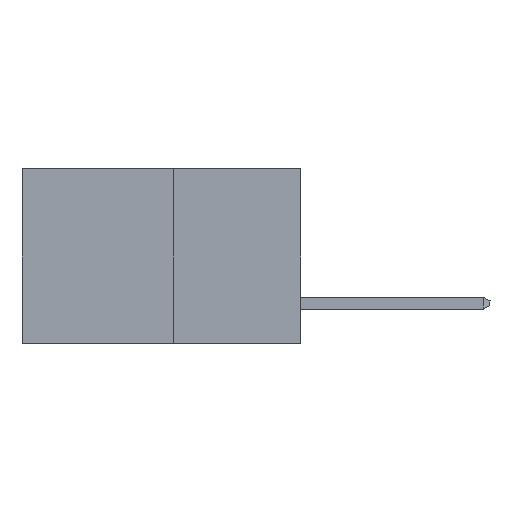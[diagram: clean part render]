
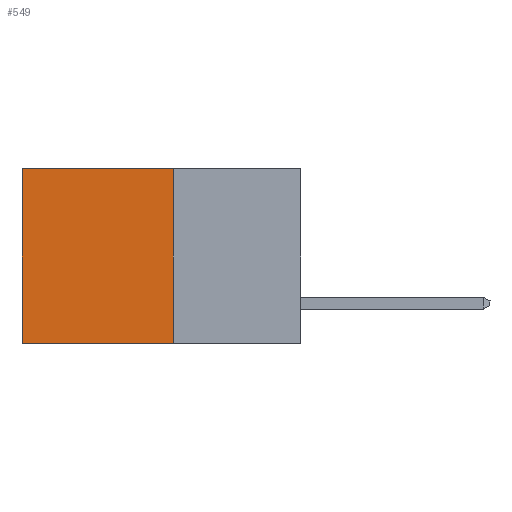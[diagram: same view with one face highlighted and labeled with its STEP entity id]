
A CAD part, left-side view. The second image highlights one B-rep face of the part: STEP entity #549.
In plain terms, the highlighted planar face has unit normal (-1, 0, 0).
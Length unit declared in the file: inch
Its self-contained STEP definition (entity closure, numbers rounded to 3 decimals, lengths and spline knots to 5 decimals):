
#549 = ADVANCED_FACE ( 'NONE', ( #6865 ), #8698, .F. ) ;
#963 = CARTESIAN_POINT ( 'NONE',  ( 0.277, 0.27, 0. ) ) ;
#969 = VECTOR ( 'NONE', #5272, 39.37008 ) ;
#1009 = EDGE_CURVE ( 'NONE', #10847, #4709, #10336, .T. ) ;
#1218 = CARTESIAN_POINT ( 'NONE',  ( 0.277, 0.27, -0.37 ) ) ;
#1883 = DIRECTION ( 'NONE',  ( 1., 0., 0. ) ) ;
#1923 = DIRECTION ( 'NONE',  ( 0., 1., 0. ) ) ;
#2955 = CARTESIAN_POINT ( 'NONE',  ( 0.277, 0.27, -0.37 ) ) ;
#3112 = CARTESIAN_POINT ( 'NONE',  ( 0.277, 0.27, -0.37 ) ) ;
#3329 = LINE ( 'NONE', #4714, #12536 ) ;
#4669 = DIRECTION ( 'NONE',  ( 0., 0., -1. ) ) ;
#4709 = VERTEX_POINT ( 'NONE', #12002 ) ;
#4714 = CARTESIAN_POINT ( 'NONE',  ( 0.277, 0.59, -0.37 ) ) ;
#5272 = DIRECTION ( 'NONE',  ( 0., 1., 0. ) ) ;
#5423 = CARTESIAN_POINT ( 'NONE',  ( 0.277, 0.59, -0.37 ) ) ;
#5936 = LINE ( 'NONE', #3112, #9105 ) ;
#6035 = VERTEX_POINT ( 'NONE', #9344 ) ;
#6489 = LINE ( 'NONE', #2955, #9983 ) ;
#6543 = AXIS2_PLACEMENT_3D ( 'NONE', #1218, #1883, #6947 ) ;
#6865 = FACE_OUTER_BOUND ( 'NONE', #13600, .T. ) ;
#6947 = DIRECTION ( 'NONE',  ( 0., 0., -1. ) ) ;
#6967 = EDGE_CURVE ( 'NONE', #4709, #12633, #3329, .T. ) ;
#8698 = PLANE ( 'NONE',  #6543 ) ;
#9105 = VECTOR ( 'NONE', #1923, 39.37008 ) ;
#9344 = CARTESIAN_POINT ( 'NONE',  ( 0.277, 0.27, -0.37 ) ) ;
#9579 = EDGE_CURVE ( 'NONE', #6035, #12633, #5936, .T. ) ;
#9983 = VECTOR ( 'NONE', #11112, 39.37008 ) ;
#10336 = LINE ( 'NONE', #12167, #969 ) ;
#10502 = ORIENTED_EDGE ( 'NONE', *, *, #6967, .T. ) ;
#10847 = VERTEX_POINT ( 'NONE', #963 ) ;
#11112 = DIRECTION ( 'NONE',  ( 0., 0., -1. ) ) ;
#11560 = ORIENTED_EDGE ( 'NONE', *, *, #14205, .F. ) ;
#12002 = CARTESIAN_POINT ( 'NONE',  ( 0.277, 0.59, 0. ) ) ;
#12167 = CARTESIAN_POINT ( 'NONE',  ( 0.277, 0.27, 0. ) ) ;
#12536 = VECTOR ( 'NONE', #4669, 39.37008 ) ;
#12633 = VERTEX_POINT ( 'NONE', #5423 ) ;
#13600 = EDGE_LOOP ( 'NONE', ( #10502, #14134, #11560, #14483 ) ) ;
#14134 = ORIENTED_EDGE ( 'NONE', *, *, #9579, .F. ) ;
#14205 = EDGE_CURVE ( 'NONE', #10847, #6035, #6489, .T. ) ;
#14483 = ORIENTED_EDGE ( 'NONE', *, *, #1009, .T. ) ;
